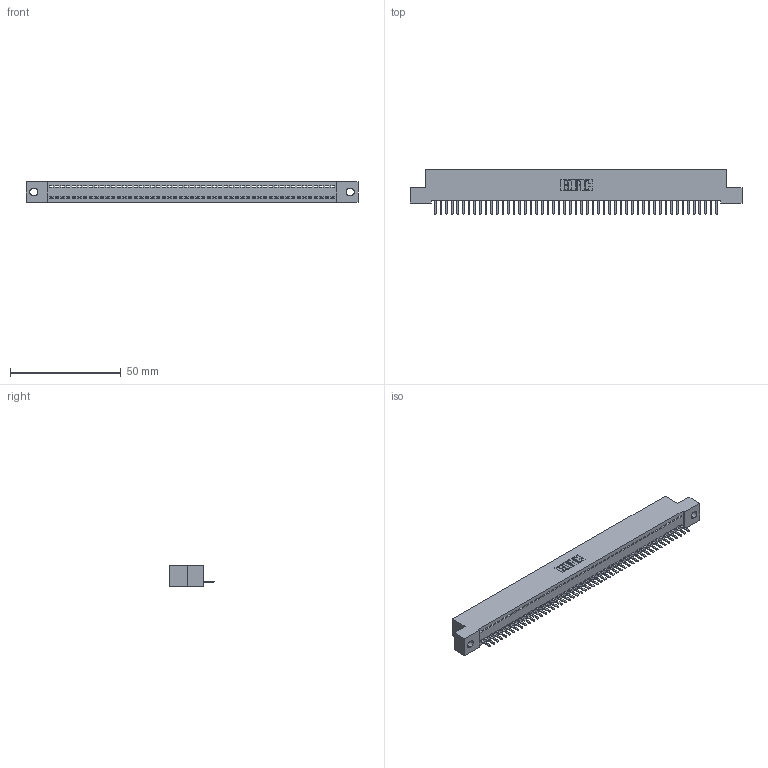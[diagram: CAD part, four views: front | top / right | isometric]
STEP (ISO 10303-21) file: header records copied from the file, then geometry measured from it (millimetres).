
FILE_DESCRIPTION (( 'STEP AP203' ), '1' );
FILE_NAME ('392-051-520-102.STEP', '2019-10-08T11:49:10', ( '' ), ( '' ), 'SwSTEP 2.0', 'SolidWorks 2016', '' );
FILE_SCHEMA (( 'CONFIG_CONTROL_DESIGN' ));
Length unit declared in the file: inch
Products named in the file (3): 342 Part_.128 Slot; 345-292-001_345-293-120; 392-051-520-102
Assembly tree (52 placements, depth 2):
  392-051-520-102
    342 Part_.128 Slot
    345-292-001_345-293-120  x51
Bounding box: 149.86 x 20.02 x 9.4 mm (x, y, z)
Volume: 12974 mm3; surface area: 18510.3 mm2
Topology: 52 solids, 52 shells, 3276 faces, 9695 edges, 6326 vertices
Faces by surface type: plane 2314, cylinder 962
Entity records: 30131 total; most frequent: CARTESIAN_POINT 5215, ORIENTED_EDGE 5190, DIRECTION 4369, EDGE_CURVE 2595, VECTOR 2463, LINE 2463, VERTEX_POINT 1726, AXIS2_PLACEMENT_3D 953
